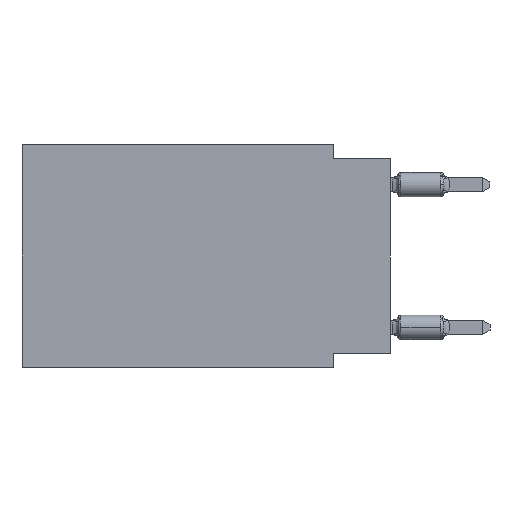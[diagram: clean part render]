
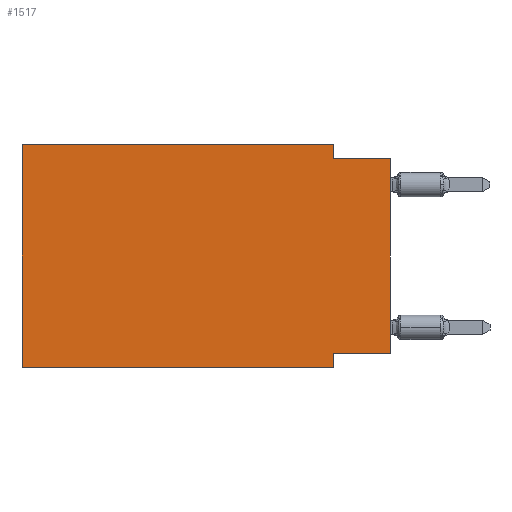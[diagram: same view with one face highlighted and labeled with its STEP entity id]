
A CAD part, left-side view. The second image highlights one B-rep face of the part: STEP entity #1517.
In plain terms, the highlighted planar face has unit normal (-1, 0, 0).
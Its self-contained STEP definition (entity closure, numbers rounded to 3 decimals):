
#657 = LINE ( 'NONE', #12858, #13148 ) ;
#750 = PLANE ( 'NONE',  #11509 ) ;
#781 = LINE ( 'NONE', #1728, #13115 ) ;
#864 = DIRECTION ( 'NONE',  ( 0., 0., -1. ) ) ;
#868 = DIRECTION ( 'NONE',  ( 0., 0., 1. ) ) ;
#871 = ORIENTED_EDGE ( 'NONE', *, *, #4064, .T. ) ;
#1045 = DIRECTION ( 'NONE',  ( 0., 0., -1. ) ) ;
#1237 = EDGE_LOOP ( 'NONE', ( #10916, #5168, #9960, #12625, #3139, #871, #7753, #5310 ) ) ;
#1517 = ADVANCED_FACE ( 'NONE', ( #4162 ), #750, .F. ) ;
#1716 = VERTEX_POINT ( 'NONE', #2213 ) ;
#1728 = CARTESIAN_POINT ( 'NONE',  ( 0., 2.54, 0. ) ) ;
#1930 = VERTEX_POINT ( 'NONE', #5520 ) ;
#1979 = VECTOR ( 'NONE', #8761, 1000. ) ;
#2213 = CARTESIAN_POINT ( 'NONE',  ( 0., 2.54, 0. ) ) ;
#2321 = LINE ( 'NONE', #6732, #12716 ) ;
#2850 = VERTEX_POINT ( 'NONE', #7854 ) ;
#3139 = ORIENTED_EDGE ( 'NONE', *, *, #5016, .F. ) ;
#3150 = CARTESIAN_POINT ( 'NONE',  ( 0., 16.383, 0. ) ) ;
#3375 = VERTEX_POINT ( 'NONE', #12442 ) ;
#3390 = CARTESIAN_POINT ( 'NONE',  ( 0., 16.383, 0. ) ) ;
#4064 = EDGE_CURVE ( 'NONE', #12255, #9966, #4316, .T. ) ;
#4162 = FACE_OUTER_BOUND ( 'NONE', #1237, .T. ) ;
#4316 = LINE ( 'NONE', #8736, #8953 ) ;
#4337 = LINE ( 'NONE', #11103, #1979 ) ;
#4833 = EDGE_CURVE ( 'NONE', #11630, #3375, #14008, .T. ) ;
#5001 = DIRECTION ( 'NONE',  ( 0., 1., 0. ) ) ;
#5016 = EDGE_CURVE ( 'NONE', #12255, #7581, #2321, .T. ) ;
#5168 = ORIENTED_EDGE ( 'NONE', *, *, #11681, .F. ) ;
#5310 = ORIENTED_EDGE ( 'NONE', *, *, #4833, .F. ) ;
#5520 = CARTESIAN_POINT ( 'NONE',  ( 0., 0., -0.635 ) ) ;
#5601 = CARTESIAN_POINT ( 'NONE',  ( 0., 16.383, 0. ) ) ;
#5640 = CARTESIAN_POINT ( 'NONE',  ( 0., 0., -0.635 ) ) ;
#5696 = VECTOR ( 'NONE', #13272, 1000. ) ;
#6435 = VECTOR ( 'NONE', #5001, 1000. ) ;
#6557 = DIRECTION ( 'NONE',  ( 0., -1., 0. ) ) ;
#6732 = CARTESIAN_POINT ( 'NONE',  ( 0., 16.383, 0. ) ) ;
#7581 = VERTEX_POINT ( 'NONE', #5601 ) ;
#7753 = ORIENTED_EDGE ( 'NONE', *, *, #9289, .F. ) ;
#7854 = CARTESIAN_POINT ( 'NONE',  ( 0., 2.54, -0.635 ) ) ;
#8521 = DIRECTION ( 'NONE',  ( 1., 0., 0. ) ) ;
#8675 = VECTOR ( 'NONE', #12048, 1000. ) ;
#8729 = EDGE_CURVE ( 'NONE', #11630, #1930, #657, .T. ) ;
#8736 = CARTESIAN_POINT ( 'NONE',  ( 0., 16.383, -9.906 ) ) ;
#8761 = DIRECTION ( 'NONE',  ( 0., 0., -1. ) ) ;
#8824 = LINE ( 'NONE', #3390, #5696 ) ;
#8953 = VECTOR ( 'NONE', #6557, 1000. ) ;
#9289 = EDGE_CURVE ( 'NONE', #3375, #9966, #4337, .T. ) ;
#9584 = CARTESIAN_POINT ( 'NONE',  ( 0., 2.54, -9.906 ) ) ;
#9942 = LINE ( 'NONE', #5640, #8675 ) ;
#9960 = ORIENTED_EDGE ( 'NONE', *, *, #12405, .F. ) ;
#9966 = VERTEX_POINT ( 'NONE', #9584 ) ;
#10916 = ORIENTED_EDGE ( 'NONE', *, *, #8729, .T. ) ;
#11103 = CARTESIAN_POINT ( 'NONE',  ( 0., 2.54, -9.906 ) ) ;
#11509 = AXIS2_PLACEMENT_3D ( 'NONE', #3150, #8521, #1045 ) ;
#11630 = VERTEX_POINT ( 'NONE', #13888 ) ;
#11681 = EDGE_CURVE ( 'NONE', #2850, #1930, #9942, .T. ) ;
#12048 = DIRECTION ( 'NONE',  ( 0., -1., 0. ) ) ;
#12255 = VERTEX_POINT ( 'NONE', #12504 ) ;
#12405 = EDGE_CURVE ( 'NONE', #1716, #2850, #781, .T. ) ;
#12442 = CARTESIAN_POINT ( 'NONE',  ( 0., 2.54, -9.271 ) ) ;
#12504 = CARTESIAN_POINT ( 'NONE',  ( 0., 16.383, -9.906 ) ) ;
#12600 = EDGE_CURVE ( 'NONE', #7581, #1716, #8824, .T. ) ;
#12625 = ORIENTED_EDGE ( 'NONE', *, *, #12600, .F. ) ;
#12716 = VECTOR ( 'NONE', #868, 1000. ) ;
#12858 = CARTESIAN_POINT ( 'NONE',  ( 0., 0., 0. ) ) ;
#13115 = VECTOR ( 'NONE', #864, 1000. ) ;
#13148 = VECTOR ( 'NONE', #14100, 1000. ) ;
#13272 = DIRECTION ( 'NONE',  ( 0., -1., 0. ) ) ;
#13877 = CARTESIAN_POINT ( 'NONE',  ( 0., 0., -9.271 ) ) ;
#13888 = CARTESIAN_POINT ( 'NONE',  ( 0., 0., -9.271 ) ) ;
#14008 = LINE ( 'NONE', #13877, #6435 ) ;
#14100 = DIRECTION ( 'NONE',  ( 0., 0., 1. ) ) ;
